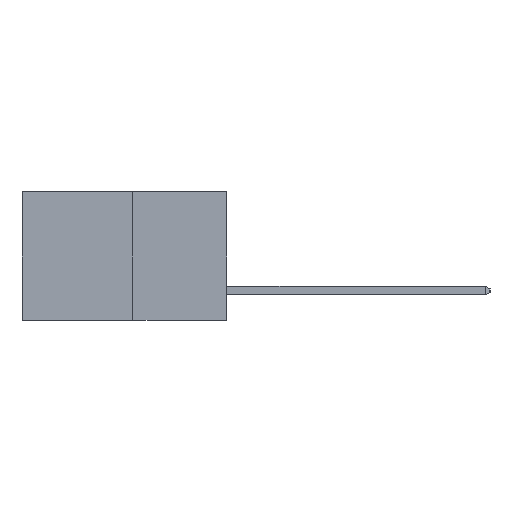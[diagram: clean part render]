
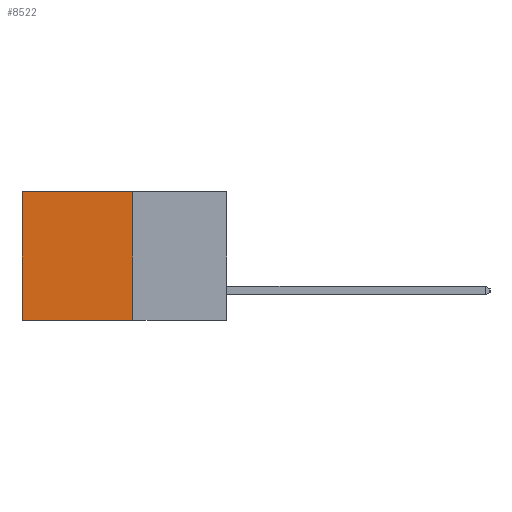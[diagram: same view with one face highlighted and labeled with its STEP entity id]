
A CAD part, left-side view. The second image highlights one B-rep face of the part: STEP entity #8522.
In plain terms, the highlighted planar face has unit normal (-1, 0, 0).
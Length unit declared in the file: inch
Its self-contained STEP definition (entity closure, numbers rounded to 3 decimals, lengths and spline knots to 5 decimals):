
#71 = VERTEX_POINT ( 'NONE', #12184 ) ;
#474 = EDGE_CURVE ( 'NONE', #71, #10383, #7402, .T. ) ;
#1069 = EDGE_CURVE ( 'NONE', #10383, #6692, #3934, .T. ) ;
#2180 = CARTESIAN_POINT ( 'NONE',  ( 0.277, 0.27, -0.37 ) ) ;
#2199 = VECTOR ( 'NONE', #5994, 39.37008 ) ;
#2631 = ORIENTED_EDGE ( 'NONE', *, *, #9234, .F. ) ;
#2913 = CARTESIAN_POINT ( 'NONE',  ( 0.277, 0.59, -0.37 ) ) ;
#3111 = FACE_OUTER_BOUND ( 'NONE', #10307, .T. ) ;
#3564 = CARTESIAN_POINT ( 'NONE',  ( 0.277, 0.59, 0. ) ) ;
#3652 = ORIENTED_EDGE ( 'NONE', *, *, #474, .T. ) ;
#3934 = LINE ( 'NONE', #11653, #5687 ) ;
#4781 = PLANE ( 'NONE',  #11059 ) ;
#5387 = EDGE_CURVE ( 'NONE', #6760, #6692, #11564, .T. ) ;
#5687 = VECTOR ( 'NONE', #9516, 39.37008 ) ;
#5876 = DIRECTION ( 'NONE',  ( 0., 0., -1. ) ) ;
#5994 = DIRECTION ( 'NONE',  ( 0., 0., -1. ) ) ;
#6252 = VECTOR ( 'NONE', #6295, 39.37008 ) ;
#6295 = DIRECTION ( 'NONE',  ( 0., 1., 0. ) ) ;
#6390 = ORIENTED_EDGE ( 'NONE', *, *, #5387, .F. ) ;
#6398 = CARTESIAN_POINT ( 'NONE',  ( 0.277, 0.27, -0.37 ) ) ;
#6642 = DIRECTION ( 'NONE',  ( 0., 1., 0. ) ) ;
#6661 = CARTESIAN_POINT ( 'NONE',  ( 0.277, 0.27, 0. ) ) ;
#6692 = VERTEX_POINT ( 'NONE', #2913 ) ;
#6760 = VERTEX_POINT ( 'NONE', #2180 ) ;
#6921 = CARTESIAN_POINT ( 'NONE',  ( 0.277, 0.27, -0.37 ) ) ;
#7402 = LINE ( 'NONE', #6661, #12653 ) ;
#8022 = LINE ( 'NONE', #9185, #2199 ) ;
#8522 = ADVANCED_FACE ( 'NONE', ( #3111 ), #4781, .F. ) ;
#9185 = CARTESIAN_POINT ( 'NONE',  ( 0.277, 0.27, -0.37 ) ) ;
#9234 = EDGE_CURVE ( 'NONE', #71, #6760, #8022, .T. ) ;
#9516 = DIRECTION ( 'NONE',  ( 0., 0., -1. ) ) ;
#9713 = ORIENTED_EDGE ( 'NONE', *, *, #1069, .T. ) ;
#10307 = EDGE_LOOP ( 'NONE', ( #9713, #6390, #2631, #3652 ) ) ;
#10383 = VERTEX_POINT ( 'NONE', #3564 ) ;
#11059 = AXIS2_PLACEMENT_3D ( 'NONE', #6921, #12240, #5876 ) ;
#11564 = LINE ( 'NONE', #6398, #6252 ) ;
#11653 = CARTESIAN_POINT ( 'NONE',  ( 0.277, 0.59, -0.37 ) ) ;
#12184 = CARTESIAN_POINT ( 'NONE',  ( 0.277, 0.27, 0. ) ) ;
#12240 = DIRECTION ( 'NONE',  ( 1., 0., 0. ) ) ;
#12653 = VECTOR ( 'NONE', #6642, 39.37008 ) ;
